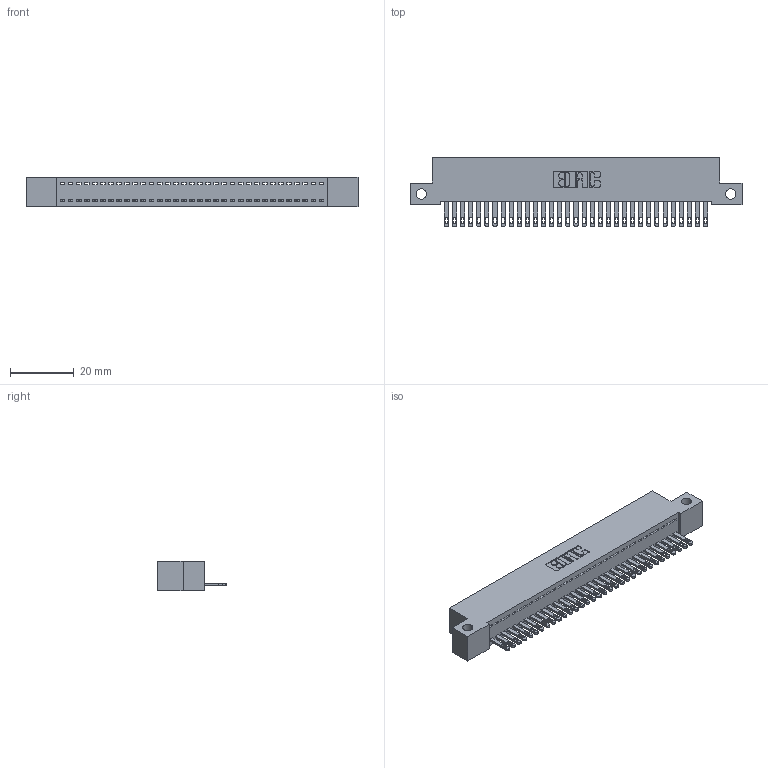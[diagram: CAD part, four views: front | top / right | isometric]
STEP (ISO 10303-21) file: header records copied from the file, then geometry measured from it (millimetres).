
FILE_DESCRIPTION (( 'STEP AP203' ), '1' );
FILE_NAME ('342-033-500-112.STEP', '2018-08-11T17:34:05', ( '' ), ( '' ), 'SwSTEP 2.0', 'SolidWorks 2016', '' );
FILE_SCHEMA (( 'CONFIG_CONTROL_DESIGN' ));
Length unit declared in the file: inch
Products named in the file (3): 342 Part_Side Mount; 345-292-001_345-293-100; 342-033-500-112
Assembly tree (34 placements, depth 2):
  342-033-500-112
    342 Part_Side Mount
    345-292-001_345-293-100  x33
Bounding box: 104.14 x 21.85 x 9.4 mm (x, y, z)
Volume: 9044.3 mm3; surface area: 13015 mm2
Topology: 34 solids, 34 shells, 1892 faces, 5843 edges, 3894 vertices
Faces by surface type: plane 1254, cylinder 638
Entity records: 21139 total; most frequent: CARTESIAN_POINT 3653, ORIENTED_EDGE 3622, DIRECTION 3101, EDGE_CURVE 1811, LINE 1679, VECTOR 1679, VERTEX_POINT 1206, AXIS2_PLACEMENT_3D 711
